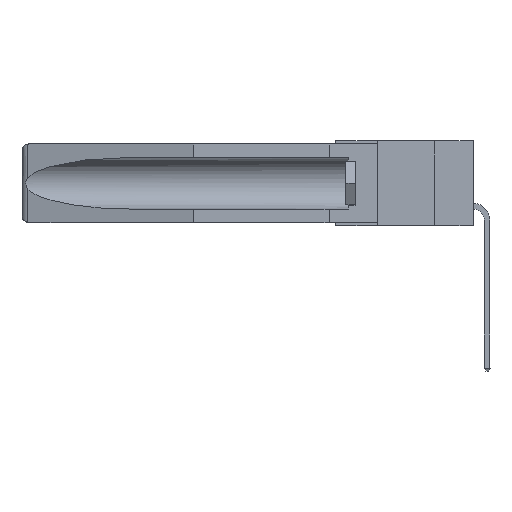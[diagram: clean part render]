
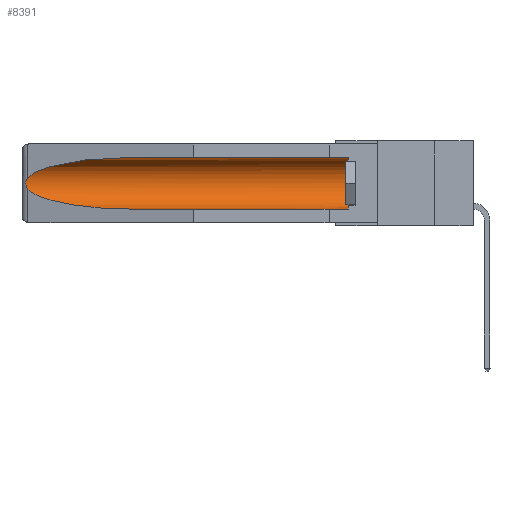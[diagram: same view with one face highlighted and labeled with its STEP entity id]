
A CAD part, left-side view. The second image highlights one B-rep face of the part: STEP entity #8391.
In plain terms, the highlighted cylindrical face has radius 2.857 mm (diameter 5.715 mm), a partial arc.
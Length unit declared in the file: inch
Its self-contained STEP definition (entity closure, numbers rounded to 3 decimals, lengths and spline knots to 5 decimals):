
#78 = ORIENTED_EDGE ( 'NONE', *, *, #18663, .F. ) ;
#813 = CARTESIAN_POINT ( 'NONE',  ( 0.155, 0.126, -0.1715 ) ) ;
#921 = DIRECTION ( 'NONE',  ( 0., 1., 0. ) ) ;
#923 = ORIENTED_EDGE ( 'NONE', *, *, #11108, .T. ) ;
#1025 = CARTESIAN_POINT ( 'NONE',  ( 0.26537, 1.52718, -0.19328 ) ) ;
#1043 = CARTESIAN_POINT ( 'NONE',  ( 0.26537, 1.52718, -0.19328 ) ) ;
#1796 = EDGE_CURVE ( 'NONE', #28964, #25872, #4377, .T. ) ;
#2181 = ORIENTED_EDGE ( 'NONE', *, *, #24603, .T. ) ;
#3129 = FACE_OUTER_BOUND ( 'NONE', #23393, .T. ) ;
#3382 = CARTESIAN_POINT ( 'NONE',  ( 0.26537, 1.52718, -0.14972 ) ) ;
#4332 = CARTESIAN_POINT ( 'NONE',  ( 0.155, 1.07973, -0.284 ) ) ;
#4360 = CARTESIAN_POINT ( 'NONE',  ( 0.26537, 1.52718, -0.14972 ) ) ;
#4377 =( BOUNDED_CURVE ( )  B_SPLINE_CURVE ( 3, ( #1043, #7887, #15093, #10098 ),
 .UNSPECIFIED., .F., .F. ) 
 B_SPLINE_CURVE_WITH_KNOTS ( ( 4, 4 ),
 ( 0.1948, 1.5708 ),
 .UNSPECIFIED. ) 
 CURVE ( )  GEOMETRIC_REPRESENTATION_ITEM ( )  RATIONAL_B_SPLINE_CURVE ( ( 1., 0.848, 0.848, 1. ) ) 
 REPRESENTATION_ITEM ( '' )  );
#4548 = CARTESIAN_POINT ( 'NONE',  ( 0.26655, 1.53094, -0.18657 ) ) ;
#5184 = CARTESIAN_POINT ( 'NONE',  ( 0.25451, 1.48313, -0.09465 ) ) ;
#5425 = LINE ( 'NONE', #6244, #29027 ) ;
#6244 = CARTESIAN_POINT ( 'NONE',  ( 0.155, -0.30754, -0.284 ) ) ;
#7489 = CARTESIAN_POINT ( 'NONE',  ( 0.26537, 1.52718, -0.14972 ) ) ;
#7624 = DIRECTION ( 'NONE',  ( 0., 0., 1. ) ) ;
#7887 = CARTESIAN_POINT ( 'NONE',  ( 0.25451, 1.48313, -0.24835 ) ) ;
#8171 =( BOUNDED_CURVE ( )  B_SPLINE_CURVE ( 3, ( #21395, #11912, #5184, #7489 ),
 .UNSPECIFIED., .F., .F. ) 
 B_SPLINE_CURVE_WITH_KNOTS ( ( 4, 4 ),
 ( 4.71239, 6.08839 ),
 .UNSPECIFIED. ) 
 CURVE ( )  GEOMETRIC_REPRESENTATION_ITEM ( )  RATIONAL_B_SPLINE_CURVE ( ( 1., 0.848, 0.848, 1. ) ) 
 REPRESENTATION_ITEM ( '' )  );
#8391 = ADVANCED_FACE ( 'NONE', ( #3129 ), #29593, .F. ) ;
#8518 = VERTEX_POINT ( 'NONE', #15024 ) ;
#8704 = VECTOR ( 'NONE', #921, 39.37008 ) ;
#10098 = CARTESIAN_POINT ( 'NONE',  ( 0.155, 1.07973, -0.284 ) ) ;
#11108 = EDGE_CURVE ( 'NONE', #8518, #15833, #24826, .T. ) ;
#11593 = ORIENTED_EDGE ( 'NONE', *, *, #1796, .T. ) ;
#11912 = CARTESIAN_POINT ( 'NONE',  ( 0.21114, 1.30732, -0.059 ) ) ;
#12310 = VERTEX_POINT ( 'NONE', #23581 ) ;
#13550 = CARTESIAN_POINT ( 'NONE',  ( 0.2673, 1.53269, -0.17917 ) ) ;
#14223 = ORIENTED_EDGE ( 'NONE', *, *, #18374, .T. ) ;
#15024 = CARTESIAN_POINT ( 'NONE',  ( 0.155, 0.126, -0.059 ) ) ;
#15093 = CARTESIAN_POINT ( 'NONE',  ( 0.21114, 1.30732, -0.284 ) ) ;
#15540 = CARTESIAN_POINT ( 'NONE',  ( 0.26537, 1.52718, -0.19328 ) ) ;
#15833 = VERTEX_POINT ( 'NONE', #25332 ) ;
#18185 = CARTESIAN_POINT ( 'NONE',  ( 0.2673, 1.5327, -0.16383 ) ) ;
#18374 = EDGE_CURVE ( 'NONE', #12310, #8518, #27951, .T. ) ;
#18546 = VERTEX_POINT ( 'NONE', #3382 ) ;
#18663 = EDGE_CURVE ( 'NONE', #12310, #25872, #5425, .T. ) ;
#18715 = ORIENTED_EDGE ( 'NONE', *, *, #26064, .T. ) ;
#19208 = B_SPLINE_CURVE_WITH_KNOTS ( 'NONE', 3,
 ( #4360, #20364, #22657, #18185, #27207, #22764, #13550, #4548, #29525, #1025 ),
 .UNSPECIFIED., .F., .F.,
 ( 4, 2, 2, 2, 4 ),
 ( 0., 0.00029, 0.00058, 0.00087, 0.00117 ),
 .UNSPECIFIED. ) ;
#20364 = CARTESIAN_POINT ( 'NONE',  ( 0.26597, 1.52961, -0.15275 ) ) ;
#21341 = DIRECTION ( 'NONE',  ( 0., 1., 0. ) ) ;
#21395 = CARTESIAN_POINT ( 'NONE',  ( 0.155, 1.07973, -0.059 ) ) ;
#22657 = CARTESIAN_POINT ( 'NONE',  ( 0.26654, 1.53092, -0.15636 ) ) ;
#22764 = CARTESIAN_POINT ( 'NONE',  ( 0.2675, 1.53308, -0.17534 ) ) ;
#23305 = AXIS2_PLACEMENT_3D ( 'NONE', #813, #23405, #23503 ) ;
#23393 = EDGE_LOOP ( 'NONE', ( #18715, #2181, #11593, #78, #14223, #923 ) ) ;
#23405 = DIRECTION ( 'NONE',  ( 0., -1., 0. ) ) ;
#23503 = DIRECTION ( 'NONE',  ( 0., 0., 1. ) ) ;
#23581 = CARTESIAN_POINT ( 'NONE',  ( 0.155, 0.126, -0.284 ) ) ;
#24603 = EDGE_CURVE ( 'NONE', #18546, #28964, #19208, .T. ) ;
#24826 = LINE ( 'NONE', #28433, #8704 ) ;
#25332 = CARTESIAN_POINT ( 'NONE',  ( 0.155, 1.07973, -0.059 ) ) ;
#25872 = VERTEX_POINT ( 'NONE', #4332 ) ;
#26064 = EDGE_CURVE ( 'NONE', #15833, #18546, #8171, .T. ) ;
#26619 = DIRECTION ( 'NONE',  ( 0., 1., 0. ) ) ;
#27207 = CARTESIAN_POINT ( 'NONE',  ( 0.2675, 1.53308, -0.16763 ) ) ;
#27951 = CIRCLE ( 'NONE', #23305, 0.1125 ) ;
#27990 = CARTESIAN_POINT ( 'NONE',  ( 0.155, -0.30754, -0.1715 ) ) ;
#28433 = CARTESIAN_POINT ( 'NONE',  ( 0.155, -0.30754, -0.059 ) ) ;
#28964 = VERTEX_POINT ( 'NONE', #15540 ) ;
#29027 = VECTOR ( 'NONE', #26619, 39.37008 ) ;
#29436 = AXIS2_PLACEMENT_3D ( 'NONE', #27990, #21341, #7624 ) ;
#29525 = CARTESIAN_POINT ( 'NONE',  ( 0.26597, 1.5296, -0.19026 ) ) ;
#29593 = CYLINDRICAL_SURFACE ( 'NONE', #29436, 0.1125 ) ;
